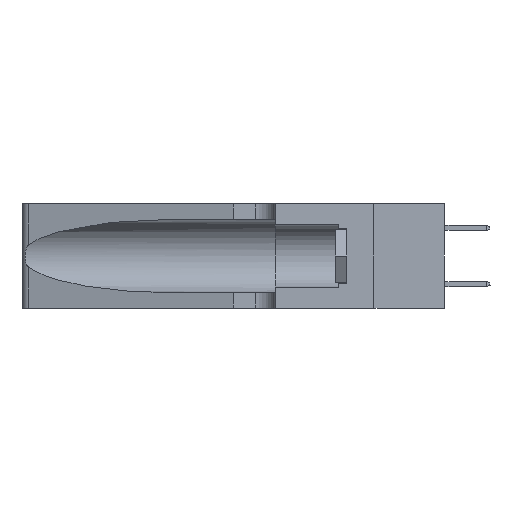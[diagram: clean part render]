
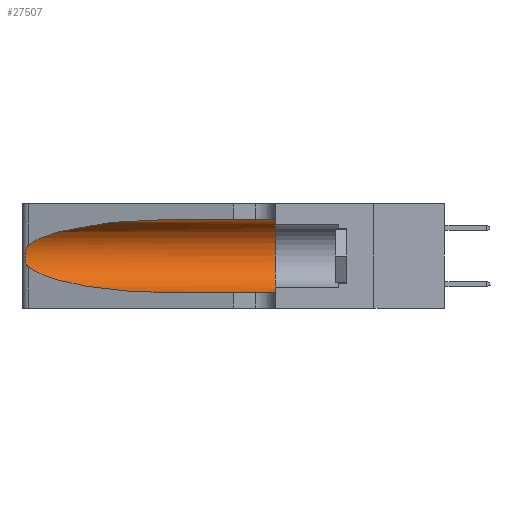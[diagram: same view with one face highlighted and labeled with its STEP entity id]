
A CAD part, left-side view. The second image highlights one B-rep face of the part: STEP entity #27507.
In plain terms, the highlighted cylindrical face has radius 3.308 mm (diameter 6.617 mm), a partial arc.
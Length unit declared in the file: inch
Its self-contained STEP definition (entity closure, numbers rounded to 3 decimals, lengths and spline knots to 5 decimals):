
#351 = CARTESIAN_POINT ( 'NONE',  ( 0.1305, 0.35, 0.31525 ) ) ;
#452 = DIRECTION ( 'NONE',  ( 0., -1., 0. ) ) ;
#1183 = CARTESIAN_POINT ( 'NONE',  ( 0.1305, 1.61858, 0.05475 ) ) ;
#1266 = CARTESIAN_POINT ( 'NONE',  ( 0.1305, 0.72297, 0.05475 ) ) ;
#1683 = VECTOR ( 'NONE', #19234, 39.37008 ) ;
#1697 = DIRECTION ( 'NONE',  ( 0., 1., 0. ) ) ;
#1837 = CARTESIAN_POINT ( 'NONE',  ( 0.25487, 1.22718, 0.22369 ) ) ;
#1943 = CARTESIAN_POINT ( 'NONE',  ( 0.25787, 1.23484, 0.2124 ) ) ;
#2247 = EDGE_CURVE ( 'NONE', #9192, #5336, #7777, .T. ) ;
#4057 = ORIENTED_EDGE ( 'NONE', *, *, #19345, .F. ) ;
#4356 = CARTESIAN_POINT ( 'NONE',  ( 0.1305, 1.61858, 0.185 ) ) ;
#4398 = CARTESIAN_POINT ( 'NONE',  ( 0.1305, 0.72297, 0.31525 ) ) ;
#4588 = CARTESIAN_POINT ( 'NONE',  ( 0.26018, 1.23835, 0.19895 ) ) ;
#4701 = EDGE_CURVE ( 'NONE', #22395, #15658, #22091, .T. ) ;
#4839 = CARTESIAN_POINT ( 'NONE',  ( 0.25487, 1.22718, 0.14631 ) ) ;
#4842 = VERTEX_POINT ( 'NONE', #29347 ) ;
#5052 = EDGE_CURVE ( 'NONE', #5977, #4842, #22260, .T. ) ;
#5336 = VERTEX_POINT ( 'NONE', #7484 ) ;
#5977 = VERTEX_POINT ( 'NONE', #20022 ) ;
#6670 = AXIS2_PLACEMENT_3D ( 'NONE', #17168, #1697, #19733 ) ;
#7188 = CARTESIAN_POINT ( 'NONE',  ( 0.26075, 1.23896, 0.178 ) ) ;
#7484 = CARTESIAN_POINT ( 'NONE',  ( 0.1305, 0.35, 0.05475 ) ) ;
#7777 = LINE ( 'NONE', #1183, #1683 ) ;
#8681 = CARTESIAN_POINT ( 'NONE',  ( 0.18966, 0.96281, 0.31525 ) ) ;
#8748 = EDGE_LOOP ( 'NONE', ( #17242, #17948, #9535, #26709, #4057, #11349 ) ) ;
#9192 = VERTEX_POINT ( 'NONE', #1266 ) ;
#9535 = ORIENTED_EDGE ( 'NONE', *, *, #26111, .T. ) ;
#9752 = CARTESIAN_POINT ( 'NONE',  ( 0.25856, 1.23593, 0.16098 ) ) ;
#9992 = CARTESIAN_POINT ( 'NONE',  ( 0.18966, 0.96281, 0.05475 ) ) ;
#10777 = FACE_OUTER_BOUND ( 'NONE', #8748, .T. ) ;
#11268 = CARTESIAN_POINT ( 'NONE',  ( 0.25487, 1.22718, 0.22369 ) ) ;
#11349 = ORIENTED_EDGE ( 'NONE', *, *, #4701, .F. ) ;
#12331 = CARTESIAN_POINT ( 'NONE',  ( 0.25639, 1.23186, 0.15144 ) ) ;
#13828 =( BOUNDED_CURVE ( )  B_SPLINE_CURVE ( 3, ( #4839, #30330, #9992, #27902 ),
 .UNSPECIFIED., .F., .F. ) 
 B_SPLINE_CURVE_WITH_KNOTS ( ( 4, 4 ),
 ( 3.44316, 4.71239 ),
 .UNSPECIFIED. ) 
 CURVE ( )  GEOMETRIC_REPRESENTATION_ITEM ( )  RATIONAL_B_SPLINE_CURVE ( ( 1., 0.87, 0.87, 1. ) ) 
 REPRESENTATION_ITEM ( '' )  );
#14940 = CARTESIAN_POINT ( 'NONE',  ( 0.25487, 1.22718, 0.14631 ) ) ;
#15658 = VERTEX_POINT ( 'NONE', #351 ) ;
#16671 = CIRCLE ( 'NONE', #6670, 0.13025 ) ;
#17168 = CARTESIAN_POINT ( 'NONE',  ( 0.1305, 0.35, 0.185 ) ) ;
#17242 = ORIENTED_EDGE ( 'NONE', *, *, #25760, .T. ) ;
#17419 = CARTESIAN_POINT ( 'NONE',  ( 0.25639, 1.23184, 0.21858 ) ) ;
#17948 = ORIENTED_EDGE ( 'NONE', *, *, #5052, .T. ) ;
#19234 = DIRECTION ( 'NONE',  ( 0., -1., 0. ) ) ;
#19345 = EDGE_CURVE ( 'NONE', #15658, #5336, #16671, .T. ) ;
#19733 = DIRECTION ( 'NONE',  ( 0., 0., 1. ) ) ;
#19789 =( BOUNDED_CURVE ( )  B_SPLINE_CURVE ( 3, ( #21461, #8681, #26598, #11268 ),
 .UNSPECIFIED., .F., .F. ) 
 B_SPLINE_CURVE_WITH_KNOTS ( ( 4, 4 ),
 ( 1.5708, 2.84003 ),
 .UNSPECIFIED. ) 
 CURVE ( )  GEOMETRIC_REPRESENTATION_ITEM ( )  RATIONAL_B_SPLINE_CURVE ( ( 1., 0.87, 0.87, 1. ) ) 
 REPRESENTATION_ITEM ( '' )  );
#19971 = CARTESIAN_POINT ( 'NONE',  ( 0.25854, 1.2359, 0.20912 ) ) ;
#20022 = CARTESIAN_POINT ( 'NONE',  ( 0.25487, 1.22718, 0.22369 ) ) ;
#21095 = CARTESIAN_POINT ( 'NONE',  ( 0.1305, 1.61858, 0.31525 ) ) ;
#21461 = CARTESIAN_POINT ( 'NONE',  ( 0.1305, 0.72297, 0.31525 ) ) ;
#22091 = LINE ( 'NONE', #21095, #28054 ) ;
#22260 = B_SPLINE_CURVE_WITH_KNOTS ( 'NONE', 3,
 ( #1837, #30104, #17419, #1943, #19971, #4588, #22575, #7188, #25121, #9752, #27667, #12331, #30208, #14940 ),
 .UNSPECIFIED., .F., .F.,
 ( 4, 2, 2, 2, 2, 2, 4 ),
 ( 0., 0.00027, 0.00053, 0.00107, 0.0016, 0.00187, 0.00214 ),
 .UNSPECIFIED. ) ;
#22331 = DIRECTION ( 'NONE',  ( 0., 0., -1. ) ) ;
#22395 = VERTEX_POINT ( 'NONE', #4398 ) ;
#22575 = CARTESIAN_POINT ( 'NONE',  ( 0.26075, 1.23896, 0.19203 ) ) ;
#24774 = DIRECTION ( 'NONE',  ( 0., -1., 0. ) ) ;
#25121 = CARTESIAN_POINT ( 'NONE',  ( 0.26017, 1.23833, 0.17102 ) ) ;
#25760 = EDGE_CURVE ( 'NONE', #22395, #5977, #19789, .T. ) ;
#26111 = EDGE_CURVE ( 'NONE', #4842, #9192, #13828, .T. ) ;
#26598 = CARTESIAN_POINT ( 'NONE',  ( 0.2373, 1.15595, 0.28018 ) ) ;
#26709 = ORIENTED_EDGE ( 'NONE', *, *, #2247, .T. ) ;
#27507 = ADVANCED_FACE ( 'NONE', ( #10777 ), #30360, .F. ) ;
#27667 = CARTESIAN_POINT ( 'NONE',  ( 0.25789, 1.23486, 0.15765 ) ) ;
#27902 = CARTESIAN_POINT ( 'NONE',  ( 0.1305, 0.72297, 0.05475 ) ) ;
#28054 = VECTOR ( 'NONE', #452, 39.37008 ) ;
#29347 = CARTESIAN_POINT ( 'NONE',  ( 0.25487, 1.22718, 0.14631 ) ) ;
#30104 = CARTESIAN_POINT ( 'NONE',  ( 0.25555, 1.22994, 0.2215 ) ) ;
#30208 = CARTESIAN_POINT ( 'NONE',  ( 0.25555, 1.22993, 0.14849 ) ) ;
#30330 = CARTESIAN_POINT ( 'NONE',  ( 0.2373, 1.15595, 0.08982 ) ) ;
#30360 = CYLINDRICAL_SURFACE ( 'NONE', #33128, 0.13025 ) ;
#33128 = AXIS2_PLACEMENT_3D ( 'NONE', #4356, #24774, #22331 ) ;
